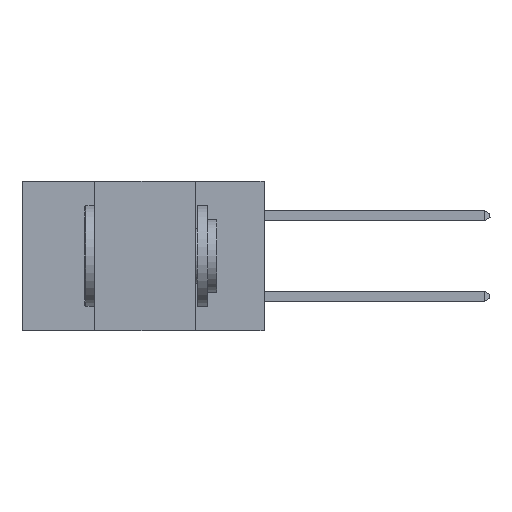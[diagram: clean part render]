
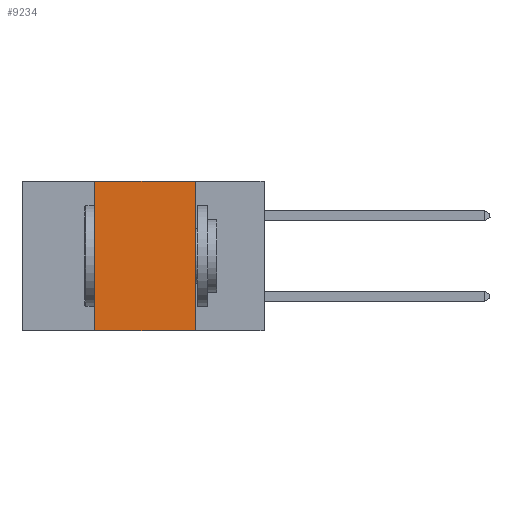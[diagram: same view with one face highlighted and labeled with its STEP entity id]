
A CAD part, left-side view. The second image highlights one B-rep face of the part: STEP entity #9234.
In plain terms, the highlighted planar face has unit normal (-1, 0, 0).
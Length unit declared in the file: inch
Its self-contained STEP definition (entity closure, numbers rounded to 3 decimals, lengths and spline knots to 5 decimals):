
#155 = VECTOR ( 'NONE', #6012, 39.37008 ) ;
#832 = DIRECTION ( 'NONE',  ( 0., -1., 0. ) ) ;
#2430 = ORIENTED_EDGE ( 'NONE', *, *, #6530, .F. ) ;
#3129 = VERTEX_POINT ( 'NONE', #6578 ) ;
#3197 = CARTESIAN_POINT ( 'NONE',  ( 0., 0.42, -0.37 ) ) ;
#3240 = PLANE ( 'NONE',  #14529 ) ;
#3970 = EDGE_CURVE ( 'NONE', #8372, #3129, #6922, .T. ) ;
#4042 = VERTEX_POINT ( 'NONE', #8433 ) ;
#5259 = ORIENTED_EDGE ( 'NONE', *, *, #3970, .F. ) ;
#6012 = DIRECTION ( 'NONE',  ( 0., -1., 0. ) ) ;
#6153 = LINE ( 'NONE', #13444, #155 ) ;
#6530 = EDGE_CURVE ( 'NONE', #3129, #4042, #18449, .T. ) ;
#6578 = CARTESIAN_POINT ( 'NONE',  ( 0., 0.42, 0. ) ) ;
#6922 = LINE ( 'NONE', #7639, #19602 ) ;
#7639 = CARTESIAN_POINT ( 'NONE',  ( 0., 0.42, 0. ) ) ;
#8372 = VERTEX_POINT ( 'NONE', #3197 ) ;
#8433 = CARTESIAN_POINT ( 'NONE',  ( 0., 0.17, 0. ) ) ;
#9230 = DIRECTION ( 'NONE',  ( 0., 0., 1. ) ) ;
#9234 = ADVANCED_FACE ( 'NONE', ( #13898 ), #3240, .F. ) ;
#10499 = ORIENTED_EDGE ( 'NONE', *, *, #12272, .F. ) ;
#11034 = DIRECTION ( 'NONE',  ( 1., 0., 0. ) ) ;
#11078 = VECTOR ( 'NONE', #832, 39.37008 ) ;
#11317 = DIRECTION ( 'NONE',  ( 0., 0., -1. ) ) ;
#11364 = CARTESIAN_POINT ( 'NONE',  ( 0., 0.6, 0. ) ) ;
#11863 = EDGE_CURVE ( 'NONE', #8372, #17171, #6153, .T. ) ;
#12272 = EDGE_CURVE ( 'NONE', #4042, #17171, #15927, .T. ) ;
#12296 = CARTESIAN_POINT ( 'NONE',  ( 0., 0.6, 0. ) ) ;
#13057 = VECTOR ( 'NONE', #11317, 39.37008 ) ;
#13444 = CARTESIAN_POINT ( 'NONE',  ( 0., 0.6, -0.37 ) ) ;
#13898 = FACE_OUTER_BOUND ( 'NONE', #14596, .T. ) ;
#14351 = ORIENTED_EDGE ( 'NONE', *, *, #11863, .T. ) ;
#14529 = AXIS2_PLACEMENT_3D ( 'NONE', #12296, #11034, #15456 ) ;
#14596 = EDGE_LOOP ( 'NONE', ( #10499, #2430, #5259, #14351 ) ) ;
#15456 = DIRECTION ( 'NONE',  ( 0., 0., -1. ) ) ;
#15927 = LINE ( 'NONE', #19070, #13057 ) ;
#17171 = VERTEX_POINT ( 'NONE', #18062 ) ;
#18062 = CARTESIAN_POINT ( 'NONE',  ( 0., 0.17, -0.37 ) ) ;
#18449 = LINE ( 'NONE', #11364, #11078 ) ;
#19070 = CARTESIAN_POINT ( 'NONE',  ( 0., 0.17, 0. ) ) ;
#19602 = VECTOR ( 'NONE', #9230, 39.37008 ) ;
